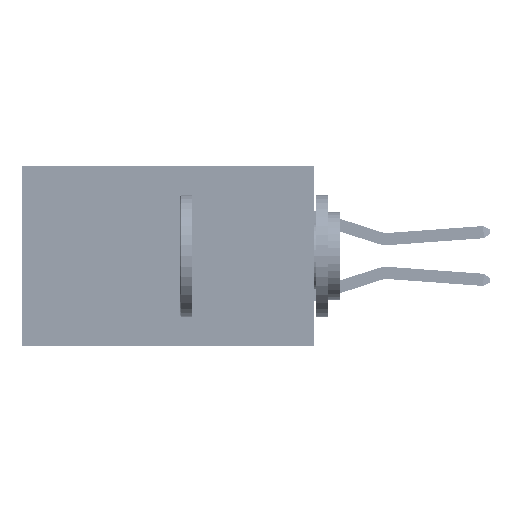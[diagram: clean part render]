
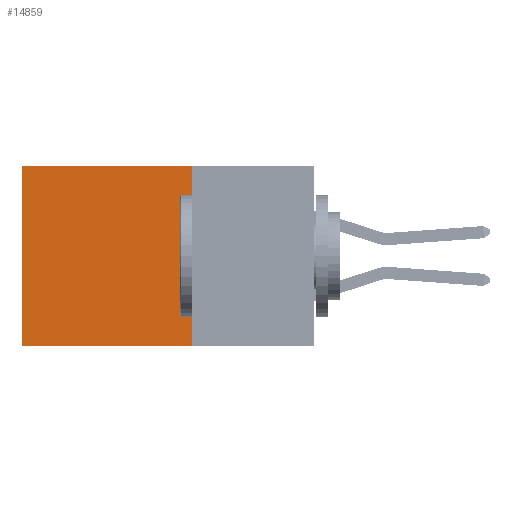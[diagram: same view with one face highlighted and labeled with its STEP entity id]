
A CAD part, left-side view. The second image highlights one B-rep face of the part: STEP entity #14859.
In plain terms, the highlighted planar face has unit normal (-1, 0, 0).
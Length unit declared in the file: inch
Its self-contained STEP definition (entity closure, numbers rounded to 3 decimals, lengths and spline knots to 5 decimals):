
#2960 = CARTESIAN_POINT ( 'NONE',  ( 0.2875, 0.25, 0. ) ) ;
#5528 = CARTESIAN_POINT ( 'NONE',  ( 0.2875, 0.6, -0.37 ) ) ;
#7513 = LINE ( 'NONE', #34632, #36260 ) ;
#7574 = ORIENTED_EDGE ( 'NONE', *, *, #34315, .F. ) ;
#9431 = EDGE_CURVE ( 'NONE', #47604, #13443, #10663, .T. ) ;
#10663 = LINE ( 'NONE', #39564, #20013 ) ;
#12320 = VERTEX_POINT ( 'NONE', #5528 ) ;
#12707 = AXIS2_PLACEMENT_3D ( 'NONE', #2960, #30564, #42165 ) ;
#12795 = ORIENTED_EDGE ( 'NONE', *, *, #37154, .T. ) ;
#12942 = ORIENTED_EDGE ( 'NONE', *, *, #39532, .F. ) ;
#13443 = VERTEX_POINT ( 'NONE', #22106 ) ;
#14859 = ADVANCED_FACE ( 'NONE', ( #32312 ), #38437, .F. ) ;
#14967 = CARTESIAN_POINT ( 'NONE',  ( 0.2875, 0.25, -0.37 ) ) ;
#16929 = EDGE_LOOP ( 'NONE', ( #12795, #7574, #12942, #49220 ) ) ;
#19000 = LINE ( 'NONE', #27926, #33379 ) ;
#20013 = VECTOR ( 'NONE', #28017, 39.37008 ) ;
#22106 = CARTESIAN_POINT ( 'NONE',  ( 0.2875, 0.6, 0. ) ) ;
#27691 = VECTOR ( 'NONE', #44646, 39.37008 ) ;
#27926 = CARTESIAN_POINT ( 'NONE',  ( 0.2875, 0.25, -0.37 ) ) ;
#28017 = DIRECTION ( 'NONE',  ( 0., 1., 0. ) ) ;
#30564 = DIRECTION ( 'NONE',  ( 1., 0., 0. ) ) ;
#32312 = FACE_OUTER_BOUND ( 'NONE', #16929, .T. ) ;
#33379 = VECTOR ( 'NONE', #47780, 39.37008 ) ;
#34275 = CARTESIAN_POINT ( 'NONE',  ( 0.2875, 0.25, 0. ) ) ;
#34315 = EDGE_CURVE ( 'NONE', #40915, #12320, #19000, .T. ) ;
#34632 = CARTESIAN_POINT ( 'NONE',  ( 0.2875, 0.25, 0. ) ) ;
#36260 = VECTOR ( 'NONE', #42039, 39.37008 ) ;
#36532 = CARTESIAN_POINT ( 'NONE',  ( 0.2875, 0.6, 0. ) ) ;
#37154 = EDGE_CURVE ( 'NONE', #13443, #12320, #47808, .T. ) ;
#38437 = PLANE ( 'NONE',  #12707 ) ;
#39532 = EDGE_CURVE ( 'NONE', #47604, #40915, #7513, .T. ) ;
#39564 = CARTESIAN_POINT ( 'NONE',  ( 0.2875, 0.25, 0. ) ) ;
#40915 = VERTEX_POINT ( 'NONE', #14967 ) ;
#42039 = DIRECTION ( 'NONE',  ( 0., 0., -1. ) ) ;
#42165 = DIRECTION ( 'NONE',  ( 0., 0., -1. ) ) ;
#44646 = DIRECTION ( 'NONE',  ( 0., 0., -1. ) ) ;
#47604 = VERTEX_POINT ( 'NONE', #34275 ) ;
#47780 = DIRECTION ( 'NONE',  ( 0., 1., 0. ) ) ;
#47808 = LINE ( 'NONE', #36532, #27691 ) ;
#49220 = ORIENTED_EDGE ( 'NONE', *, *, #9431, .T. ) ;
